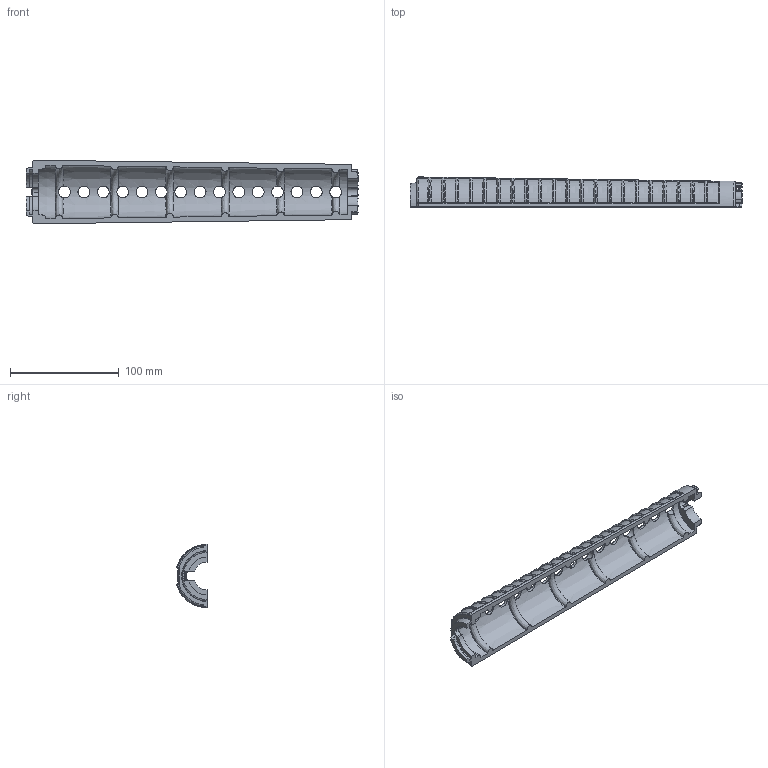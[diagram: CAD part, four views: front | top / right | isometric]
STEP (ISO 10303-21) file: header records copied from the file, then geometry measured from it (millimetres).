
FILE_DESCRIPTION (( 'STEP AP214' ), '1' );
FILE_NAME ('AR15-hand guard half.STEP', '2013-06-18T15:30:03', ( 'Asher' ), ( '' ), 'SwSTEP 2.0', 'SolidWorks 2013', '' );
FILE_SCHEMA (( 'AUTOMOTIVE_DESIGN' ));
Length unit declared in the file: millimetre
Products named in the file (1): AR15-hand guard half
Bounding box: 304.8 x 27.59 x 58.39 mm (x, y, z)
Volume: 87545.5 mm3; surface area: 54794.3 mm2
Topology: 1 solids, 1 shells, 1490 faces, 3879 edges, 2167 vertices
Faces by surface type: bspline 971, plane 329, cylinder 131, cone 57, torus 2
Entity records: 80967 total; most frequent: CARTESIAN_POINT 54270, ORIENTED_EDGE 7348, EDGE_CURVE 3674, DIRECTION 2712, B_SPLINE_CURVE_WITH_KNOTS 2493, VERTEX_POINT 2167, EDGE_LOOP 1501, ADVANCED_FACE 1490
